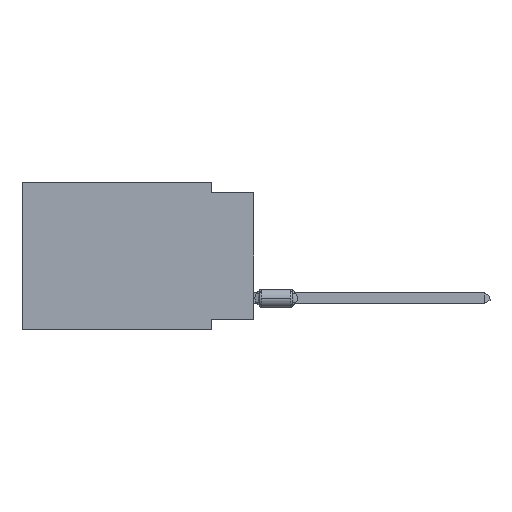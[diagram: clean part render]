
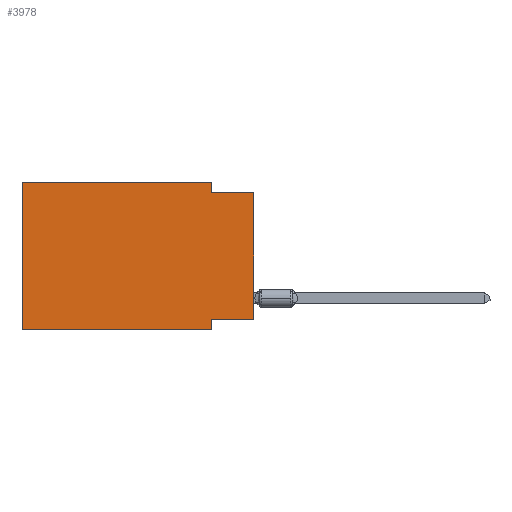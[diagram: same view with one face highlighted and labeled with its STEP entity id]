
A CAD part, left-side view. The second image highlights one B-rep face of the part: STEP entity #3978.
In plain terms, the highlighted planar face has unit normal (-1, 0, 0).
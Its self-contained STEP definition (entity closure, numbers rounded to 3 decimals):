
#292 = EDGE_CURVE ( 'NONE', #13788, #7290, #355, .T. ) ;
#324 = CARTESIAN_POINT ( 'NONE',  ( 0., 13.97, -8.89 ) ) ;
#344 = LINE ( 'NONE', #5916, #14747 ) ;
#355 = LINE ( 'NONE', #4733, #9650 ) ;
#422 = EDGE_CURVE ( 'NONE', #14965, #3553, #6474, .T. ) ;
#1200 = CARTESIAN_POINT ( 'NONE',  ( 0., 2.54, -8.89 ) ) ;
#1357 = VECTOR ( 'NONE', #16544, 1000. ) ;
#1598 = CARTESIAN_POINT ( 'NONE',  ( 0., 0., -8.255 ) ) ;
#1692 = VECTOR ( 'NONE', #7150, 1000. ) ;
#1966 = CARTESIAN_POINT ( 'NONE',  ( 0., 13.97, 0. ) ) ;
#3059 = AXIS2_PLACEMENT_3D ( 'NONE', #1966, #13290, #13205 ) ;
#3092 = VERTEX_POINT ( 'NONE', #1200 ) ;
#3158 = FACE_OUTER_BOUND ( 'NONE', #15256, .T. ) ;
#3531 = ORIENTED_EDGE ( 'NONE', *, *, #292, .F. ) ;
#3553 = VERTEX_POINT ( 'NONE', #16528 ) ;
#3705 = VERTEX_POINT ( 'NONE', #14618 ) ;
#3978 = ADVANCED_FACE ( 'NONE', ( #3158 ), #5981, .F. ) ;
#4130 = LINE ( 'NONE', #5232, #15095 ) ;
#4301 = LINE ( 'NONE', #6872, #1357 ) ;
#4364 = ORIENTED_EDGE ( 'NONE', *, *, #8218, .F. ) ;
#4543 = DIRECTION ( 'NONE',  ( 0., 0., -1. ) ) ;
#4733 = CARTESIAN_POINT ( 'NONE',  ( 0., 13.97, 0. ) ) ;
#5232 = CARTESIAN_POINT ( 'NONE',  ( 0., 13.97, 0. ) ) ;
#5916 = CARTESIAN_POINT ( 'NONE',  ( 0., 2.54, 0. ) ) ;
#5981 = PLANE ( 'NONE',  #3059 ) ;
#6419 = LINE ( 'NONE', #14565, #8003 ) ;
#6474 = LINE ( 'NONE', #12038, #12573 ) ;
#6574 = ORIENTED_EDGE ( 'NONE', *, *, #422, .T. ) ;
#6872 = CARTESIAN_POINT ( 'NONE',  ( 0., 0., -8.255 ) ) ;
#7150 = DIRECTION ( 'NONE',  ( 0., 0., -1. ) ) ;
#7290 = VERTEX_POINT ( 'NONE', #11693 ) ;
#7885 = ORIENTED_EDGE ( 'NONE', *, *, #13793, .F. ) ;
#8003 = VECTOR ( 'NONE', #17638, 1000. ) ;
#8080 = DIRECTION ( 'NONE',  ( 0., 0., 1. ) ) ;
#8187 = ORIENTED_EDGE ( 'NONE', *, *, #12683, .F. ) ;
#8218 = EDGE_CURVE ( 'NONE', #14966, #13788, #4130, .T. ) ;
#8473 = VECTOR ( 'NONE', #17114, 1000. ) ;
#9535 = LINE ( 'NONE', #13910, #1692 ) ;
#9605 = CARTESIAN_POINT ( 'NONE',  ( 0., 2.54, -0.635 ) ) ;
#9650 = VECTOR ( 'NONE', #15881, 1000. ) ;
#9735 = VERTEX_POINT ( 'NONE', #9605 ) ;
#10319 = EDGE_CURVE ( 'NONE', #14966, #3092, #14737, .T. ) ;
#10818 = ORIENTED_EDGE ( 'NONE', *, *, #10319, .T. ) ;
#11693 = CARTESIAN_POINT ( 'NONE',  ( 0., 2.54, 0. ) ) ;
#12038 = CARTESIAN_POINT ( 'NONE',  ( 0., 0., 0. ) ) ;
#12573 = VECTOR ( 'NONE', #17601, 1000. ) ;
#12683 = EDGE_CURVE ( 'NONE', #9735, #3553, #6419, .T. ) ;
#13057 = CARTESIAN_POINT ( 'NONE',  ( 0., 13.97, 0. ) ) ;
#13205 = DIRECTION ( 'NONE',  ( 0., 0., -1. ) ) ;
#13290 = DIRECTION ( 'NONE',  ( 1., 0., 0. ) ) ;
#13788 = VERTEX_POINT ( 'NONE', #13057 ) ;
#13793 = EDGE_CURVE ( 'NONE', #7290, #9735, #344, .T. ) ;
#13910 = CARTESIAN_POINT ( 'NONE',  ( 0., 2.54, -8.89 ) ) ;
#14565 = CARTESIAN_POINT ( 'NONE',  ( 0., 0., -0.635 ) ) ;
#14618 = CARTESIAN_POINT ( 'NONE',  ( 0., 2.54, -8.255 ) ) ;
#14737 = LINE ( 'NONE', #17209, #8473 ) ;
#14747 = VECTOR ( 'NONE', #4543, 1000. ) ;
#14965 = VERTEX_POINT ( 'NONE', #1598 ) ;
#14966 = VERTEX_POINT ( 'NONE', #324 ) ;
#15095 = VECTOR ( 'NONE', #8080, 1000. ) ;
#15256 = EDGE_LOOP ( 'NONE', ( #6574, #8187, #7885, #3531, #4364, #10818, #18023, #17714 ) ) ;
#15881 = DIRECTION ( 'NONE',  ( 0., -1., 0. ) ) ;
#16528 = CARTESIAN_POINT ( 'NONE',  ( 0., 0., -0.635 ) ) ;
#16544 = DIRECTION ( 'NONE',  ( 0., 1., 0. ) ) ;
#16827 = EDGE_CURVE ( 'NONE', #14965, #3705, #4301, .T. ) ;
#17114 = DIRECTION ( 'NONE',  ( 0., -1., 0. ) ) ;
#17209 = CARTESIAN_POINT ( 'NONE',  ( 0., 13.97, -8.89 ) ) ;
#17601 = DIRECTION ( 'NONE',  ( 0., 0., 1. ) ) ;
#17638 = DIRECTION ( 'NONE',  ( 0., -1., 0. ) ) ;
#17714 = ORIENTED_EDGE ( 'NONE', *, *, #16827, .F. ) ;
#17987 = EDGE_CURVE ( 'NONE', #3705, #3092, #9535, .T. ) ;
#18023 = ORIENTED_EDGE ( 'NONE', *, *, #17987, .F. ) ;
